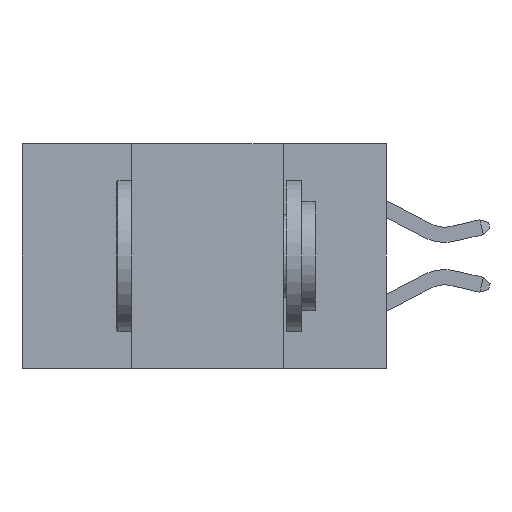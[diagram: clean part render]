
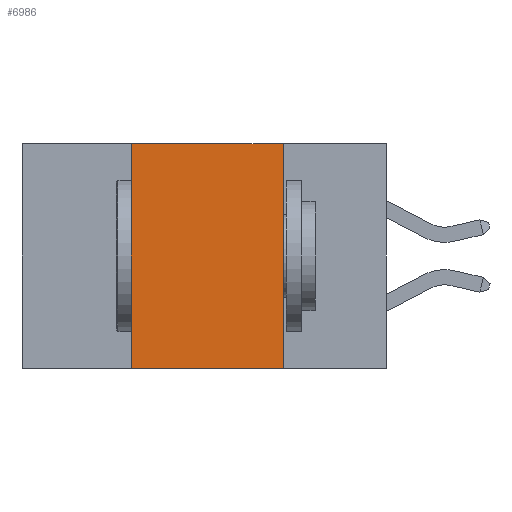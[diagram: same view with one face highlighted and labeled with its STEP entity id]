
A CAD part, left-side view. The second image highlights one B-rep face of the part: STEP entity #6986.
In plain terms, the highlighted planar face has unit normal (-1, 0, 0).
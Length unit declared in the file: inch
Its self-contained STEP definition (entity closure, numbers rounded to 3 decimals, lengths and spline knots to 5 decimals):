
#66 = LINE ( 'NONE', #3690, #12995 ) ;
#114 = EDGE_LOOP ( 'NONE', ( #11031, #6101, #2078, #10383 ) ) ;
#157 = EDGE_CURVE ( 'NONE', #8955, #5466, #66, .T. ) ;
#734 = DIRECTION ( 'NONE',  ( 0., 0., 1. ) ) ;
#2078 = ORIENTED_EDGE ( 'NONE', *, *, #10070, .F. ) ;
#2561 = FACE_OUTER_BOUND ( 'NONE', #114, .T. ) ;
#2962 = LINE ( 'NONE', #8966, #13111 ) ;
#3351 = CARTESIAN_POINT ( 'NONE',  ( 0., 0.6, -0.37 ) ) ;
#3690 = CARTESIAN_POINT ( 'NONE',  ( 0., 0.17, 0. ) ) ;
#3982 = EDGE_CURVE ( 'NONE', #11476, #8955, #6645, .T. ) ;
#4208 = CARTESIAN_POINT ( 'NONE',  ( 0., 0.17, 0. ) ) ;
#4423 = DIRECTION ( 'NONE',  ( 0., -1., 0. ) ) ;
#4735 = DIRECTION ( 'NONE',  ( 0., 0., -1. ) ) ;
#5366 = CARTESIAN_POINT ( 'NONE',  ( 0., 0.6, 0. ) ) ;
#5466 = VERTEX_POINT ( 'NONE', #10830 ) ;
#5861 = DIRECTION ( 'NONE',  ( 1., 0., 0. ) ) ;
#6101 = ORIENTED_EDGE ( 'NONE', *, *, #3982, .F. ) ;
#6332 = AXIS2_PLACEMENT_3D ( 'NONE', #12170, #5861, #4735 ) ;
#6645 = LINE ( 'NONE', #5366, #7299 ) ;
#6820 = DIRECTION ( 'NONE',  ( 0., 0., -1. ) ) ;
#6986 = ADVANCED_FACE ( 'NONE', ( #2561 ), #11030, .F. ) ;
#7113 = CARTESIAN_POINT ( 'NONE',  ( 0., 0.42, -0.37 ) ) ;
#7191 = VERTEX_POINT ( 'NONE', #7113 ) ;
#7299 = VECTOR ( 'NONE', #11768, 39.37008 ) ;
#8210 = VECTOR ( 'NONE', #4423, 39.37008 ) ;
#8257 = CARTESIAN_POINT ( 'NONE',  ( 0., 0.42, 0. ) ) ;
#8955 = VERTEX_POINT ( 'NONE', #4208 ) ;
#8966 = CARTESIAN_POINT ( 'NONE',  ( 0., 0.42, 0. ) ) ;
#9051 = LINE ( 'NONE', #3351, #8210 ) ;
#9199 = EDGE_CURVE ( 'NONE', #7191, #5466, #9051, .T. ) ;
#10070 = EDGE_CURVE ( 'NONE', #7191, #11476, #2962, .T. ) ;
#10383 = ORIENTED_EDGE ( 'NONE', *, *, #9199, .T. ) ;
#10830 = CARTESIAN_POINT ( 'NONE',  ( 0., 0.17, -0.37 ) ) ;
#11030 = PLANE ( 'NONE',  #6332 ) ;
#11031 = ORIENTED_EDGE ( 'NONE', *, *, #157, .F. ) ;
#11476 = VERTEX_POINT ( 'NONE', #8257 ) ;
#11768 = DIRECTION ( 'NONE',  ( 0., -1., 0. ) ) ;
#12170 = CARTESIAN_POINT ( 'NONE',  ( 0., 0.6, 0. ) ) ;
#12995 = VECTOR ( 'NONE', #6820, 39.37008 ) ;
#13111 = VECTOR ( 'NONE', #734, 39.37008 ) ;
